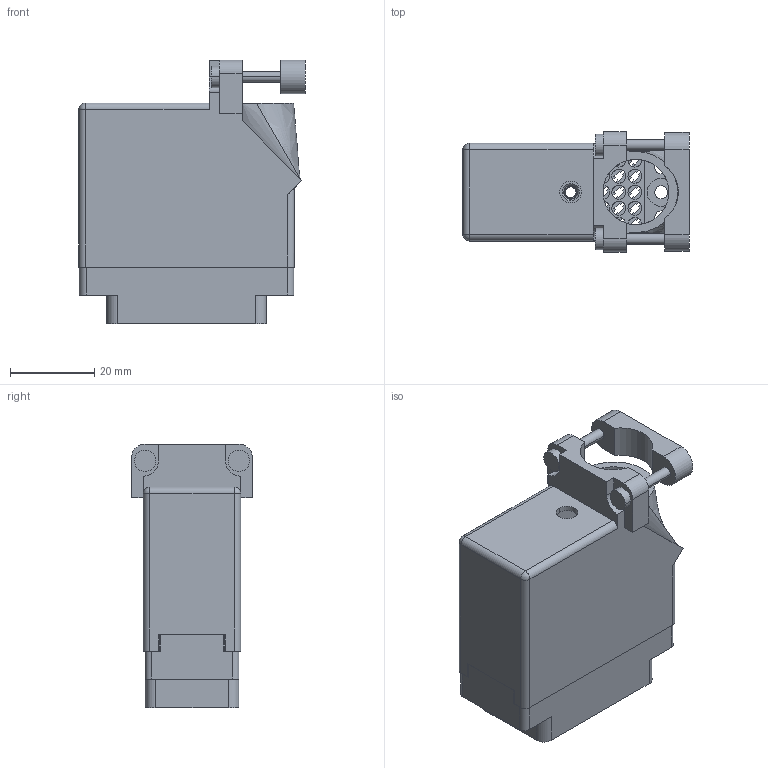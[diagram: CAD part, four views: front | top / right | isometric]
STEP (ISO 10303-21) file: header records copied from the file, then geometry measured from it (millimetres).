
FILE_DESCRIPTION (( 'STEP AP203' ), '1' );
FILE_NAME ('519-036-000-336.STEP', '2020-03-02T21:28:46', ( '' ), ( '' ), 'SwSTEP 2.0', 'SolidWorks 2016', '' );
FILE_SCHEMA (( 'CONFIG_CONTROL_DESIGN' ));
Length unit declared in the file: inch
Products named in the file (4): 516-230-001_Plastic - 038 Top Entry - Large Clamp; 519 Plug Insulator_036; 516-252-035-100_516-252-035-100; 519-036-000-336
Assembly tree (3 placements, depth 2):
  519-036-000-336
    519 Plug Insulator_036
    516-252-035-100_516-252-035-100
    516-230-001_Plastic - 038 Top Entry - Large Clamp
Bounding box: 53.62 x 28.57 x 62.48 mm (x, y, z)
Volume: 20282.9 mm3; surface area: 26105.4 mm2
Topology: 3 solids, 3 shells, 989 faces, 2863 edges, 1902 vertices
Faces by surface type: plane 671, cylinder 295, cone 12, bspline 9, sphere 2
Entity records: 35502 total; most frequent: CARTESIAN_POINT 8297, ORIENTED_EDGE 5722, DIRECTION 5500, EDGE_CURVE 2861, VECTOR 2086, LINE 2086, VERTEX_POINT 1902, AXIS2_PLACEMENT_3D 1707
